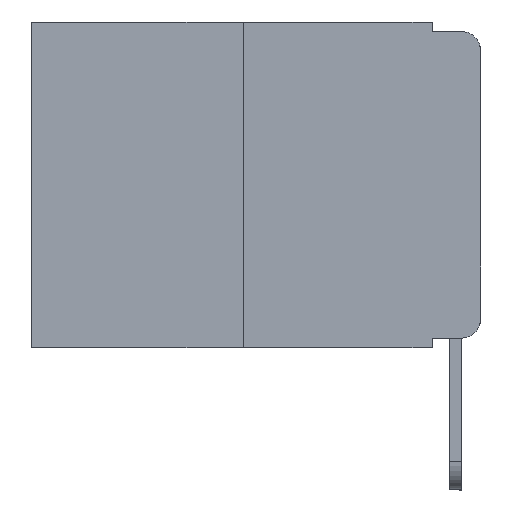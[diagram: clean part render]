
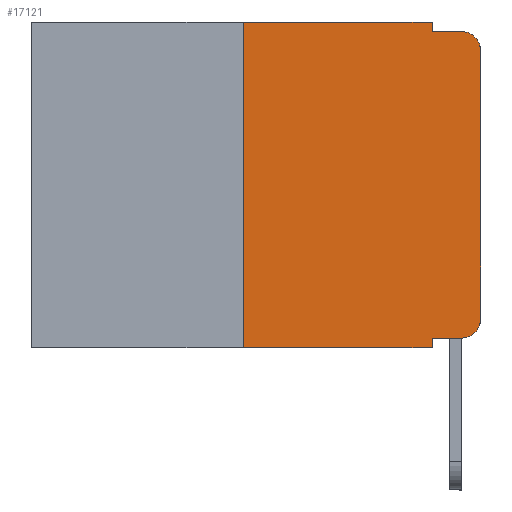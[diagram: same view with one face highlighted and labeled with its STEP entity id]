
A CAD part, left-side view. The second image highlights one B-rep face of the part: STEP entity #17121.
In plain terms, the highlighted planar face has unit normal (-1, 0, 0).
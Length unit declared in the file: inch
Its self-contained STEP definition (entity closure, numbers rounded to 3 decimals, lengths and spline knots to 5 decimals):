
#34 = CARTESIAN_POINT ( 'NONE',  ( 0., 0.051, -0.343 ) ) ;
#122 = VECTOR ( 'NONE', #20681, 39.37008 ) ;
#307 = CIRCLE ( 'NONE', #2005, 0.02 ) ;
#400 = VERTEX_POINT ( 'NONE', #13444 ) ;
#641 = DIRECTION ( 'NONE',  ( 1., 0., 0. ) ) ;
#669 = CARTESIAN_POINT ( 'NONE',  ( 0., 0., 0. ) ) ;
#778 = DIRECTION ( 'NONE',  ( -1., 0., 0. ) ) ;
#788 = VECTOR ( 'NONE', #19970, 39.37008 ) ;
#1073 = ORIENTED_EDGE ( 'NONE', *, *, #16874, .T. ) ;
#1151 = LINE ( 'NONE', #10519, #10839 ) ;
#1236 = LINE ( 'NONE', #13797, #15372 ) ;
#1729 = ORIENTED_EDGE ( 'NONE', *, *, #19950, .F. ) ;
#1767 = VERTEX_POINT ( 'NONE', #13306 ) ;
#2005 = AXIS2_PLACEMENT_3D ( 'NONE', #9139, #18912, #5858 ) ;
#2014 = AXIS2_PLACEMENT_3D ( 'NONE', #16812, #778, #12165 ) ;
#2019 = EDGE_CURVE ( 'NONE', #12752, #1767, #1236, .T. ) ;
#2473 = DIRECTION ( 'NONE',  ( 0., 0., -1. ) ) ;
#2482 = VECTOR ( 'NONE', #4274, 39.37008 ) ;
#2996 = ORIENTED_EDGE ( 'NONE', *, *, #7500, .T. ) ;
#3445 = CARTESIAN_POINT ( 'NONE',  ( 0., 0.051, 0. ) ) ;
#3903 = DIRECTION ( 'NONE',  ( 0., 0., -1. ) ) ;
#3974 = EDGE_CURVE ( 'NONE', #12623, #18718, #6800, .T. ) ;
#4270 = EDGE_LOOP ( 'NONE', ( #9207, #19030, #14108, #1729, #8233, #8752, #1073, #6846, #6411, #2996 ) ) ;
#4274 = DIRECTION ( 'NONE',  ( 0., -1., 0. ) ) ;
#4864 = CARTESIAN_POINT ( 'NONE',  ( 0., 0.473, -0.343 ) ) ;
#5434 = VECTOR ( 'NONE', #10051, 39.37008 ) ;
#5647 = CARTESIAN_POINT ( 'NONE',  ( 0., 0.051, -0.333 ) ) ;
#5858 = DIRECTION ( 'NONE',  ( 0., 0., -1. ) ) ;
#5911 = VECTOR ( 'NONE', #12884, 39.37008 ) ;
#6411 = ORIENTED_EDGE ( 'NONE', *, *, #13245, .T. ) ;
#6769 = LINE ( 'NONE', #4864, #5911 ) ;
#6800 = LINE ( 'NONE', #669, #5434 ) ;
#6842 = CARTESIAN_POINT ( 'NONE',  ( 0., 0., -0.313 ) ) ;
#6846 = ORIENTED_EDGE ( 'NONE', *, *, #12947, .F. ) ;
#7225 = CARTESIAN_POINT ( 'NONE',  ( 0., 0., -0.03 ) ) ;
#7500 = EDGE_CURVE ( 'NONE', #19410, #12623, #307, .T. ) ;
#7668 = EDGE_CURVE ( 'NONE', #18718, #1767, #9419, .T. ) ;
#7980 = LINE ( 'NONE', #3445, #788 ) ;
#8233 = ORIENTED_EDGE ( 'NONE', *, *, #13355, .F. ) ;
#8752 = ORIENTED_EDGE ( 'NONE', *, *, #12184, .F. ) ;
#9114 = LINE ( 'NONE', #10779, #11699 ) ;
#9139 = CARTESIAN_POINT ( 'NONE',  ( 0., 0.02, -0.313 ) ) ;
#9207 = ORIENTED_EDGE ( 'NONE', *, *, #3974, .T. ) ;
#9336 = LINE ( 'NONE', #20794, #122 ) ;
#9419 = CIRCLE ( 'NONE', #2014, 0.02 ) ;
#10051 = DIRECTION ( 'NONE',  ( 0., 0., 1. ) ) ;
#10519 = CARTESIAN_POINT ( 'NONE',  ( 0., 0.25, 0. ) ) ;
#10779 = CARTESIAN_POINT ( 'NONE',  ( 0., 0.051, 0. ) ) ;
#10839 = VECTOR ( 'NONE', #18527, 39.37008 ) ;
#11505 = VERTEX_POINT ( 'NONE', #18045 ) ;
#11699 = VECTOR ( 'NONE', #2473, 39.37008 ) ;
#12125 = CARTESIAN_POINT ( 'NONE',  ( 0., 0.473, 0. ) ) ;
#12165 = DIRECTION ( 'NONE',  ( 0., 0., -1. ) ) ;
#12184 = EDGE_CURVE ( 'NONE', #16333, #400, #1151, .T. ) ;
#12310 = DIRECTION ( 'NONE',  ( 0., -1., 0. ) ) ;
#12623 = VERTEX_POINT ( 'NONE', #6842 ) ;
#12752 = VERTEX_POINT ( 'NONE', #20406 ) ;
#12884 = DIRECTION ( 'NONE',  ( 0., -1., 0. ) ) ;
#12947 = EDGE_CURVE ( 'NONE', #16727, #17656, #7980, .T. ) ;
#13245 = EDGE_CURVE ( 'NONE', #16727, #19410, #18692, .T. ) ;
#13306 = CARTESIAN_POINT ( 'NONE',  ( 0., 0.02, -0.01 ) ) ;
#13355 = EDGE_CURVE ( 'NONE', #400, #11505, #9336, .T. ) ;
#13444 = CARTESIAN_POINT ( 'NONE',  ( 0., 0.25, 0. ) ) ;
#13678 = AXIS2_PLACEMENT_3D ( 'NONE', #12125, #641, #3903 ) ;
#13797 = CARTESIAN_POINT ( 'NONE',  ( 0., 0.051, -0.01 ) ) ;
#14108 = ORIENTED_EDGE ( 'NONE', *, *, #2019, .F. ) ;
#14245 = CARTESIAN_POINT ( 'NONE',  ( 0., 0.051, -0.333 ) ) ;
#15074 = FACE_OUTER_BOUND ( 'NONE', #4270, .T. ) ;
#15372 = VECTOR ( 'NONE', #12310, 39.37008 ) ;
#16333 = VERTEX_POINT ( 'NONE', #17631 ) ;
#16727 = VERTEX_POINT ( 'NONE', #14245 ) ;
#16812 = CARTESIAN_POINT ( 'NONE',  ( 0., 0.02, -0.03 ) ) ;
#16874 = EDGE_CURVE ( 'NONE', #16333, #17656, #6769, .T. ) ;
#17121 = ADVANCED_FACE ( 'NONE', ( #15074 ), #18326, .F. ) ;
#17631 = CARTESIAN_POINT ( 'NONE',  ( 0., 0.25, -0.343 ) ) ;
#17656 = VERTEX_POINT ( 'NONE', #34 ) ;
#18045 = CARTESIAN_POINT ( 'NONE',  ( 0., 0.051, 0. ) ) ;
#18326 = PLANE ( 'NONE',  #13678 ) ;
#18397 = CARTESIAN_POINT ( 'NONE',  ( 0., 0.02, -0.333 ) ) ;
#18527 = DIRECTION ( 'NONE',  ( 0., 0., 1. ) ) ;
#18692 = LINE ( 'NONE', #5647, #2482 ) ;
#18718 = VERTEX_POINT ( 'NONE', #7225 ) ;
#18912 = DIRECTION ( 'NONE',  ( -1., 0., 0. ) ) ;
#19030 = ORIENTED_EDGE ( 'NONE', *, *, #7668, .T. ) ;
#19410 = VERTEX_POINT ( 'NONE', #18397 ) ;
#19950 = EDGE_CURVE ( 'NONE', #11505, #12752, #9114, .T. ) ;
#19970 = DIRECTION ( 'NONE',  ( 0., 0., -1. ) ) ;
#20406 = CARTESIAN_POINT ( 'NONE',  ( 0., 0.051, -0.01 ) ) ;
#20681 = DIRECTION ( 'NONE',  ( 0., -1., 0. ) ) ;
#20794 = CARTESIAN_POINT ( 'NONE',  ( 0., 0.473, 0. ) ) ;
